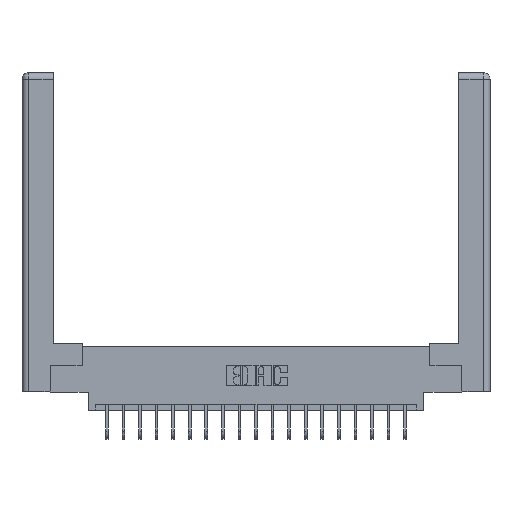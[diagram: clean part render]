
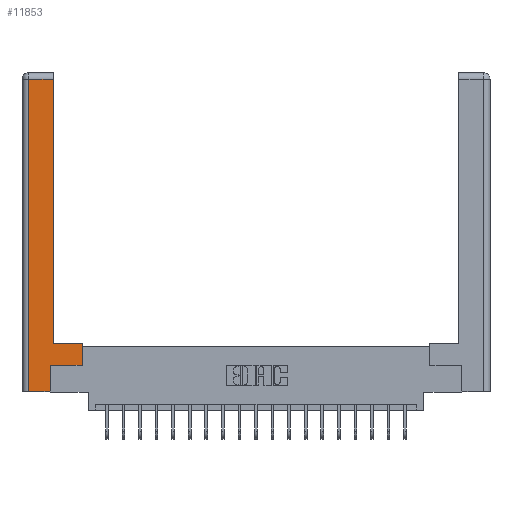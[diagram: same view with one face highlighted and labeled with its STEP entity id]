
A CAD part, top view. The second image highlights one B-rep face of the part: STEP entity #11853.
In plain terms, the highlighted planar face has unit normal (0, 0, 1).
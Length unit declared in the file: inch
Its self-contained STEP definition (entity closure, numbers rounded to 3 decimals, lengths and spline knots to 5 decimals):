
#339 = ORIENTED_EDGE ( 'NONE', *, *, #3760, .T. ) ;
#379 = ORIENTED_EDGE ( 'NONE', *, *, #7342, .T. ) ;
#838 = LINE ( 'NONE', #19871, #16722 ) ;
#1126 = DIRECTION ( 'NONE',  ( 0., 1., 0. ) ) ;
#1368 = VECTOR ( 'NONE', #1126, 39.37008 ) ;
#1410 = CARTESIAN_POINT ( 'NONE',  ( 0.265, 0., 0. ) ) ;
#1570 = DIRECTION ( 'NONE',  ( 0., -1., 0. ) ) ;
#1573 = DIRECTION ( 'NONE',  ( 0., 0., -1. ) ) ;
#1800 = CARTESIAN_POINT ( 'NONE',  ( 0.295, 2.94, 0. ) ) ;
#2307 = VECTOR ( 'NONE', #7888, 39.37008 ) ;
#2729 = VERTEX_POINT ( 'NONE', #1410 ) ;
#2953 = PLANE ( 'NONE',  #9144 ) ;
#3264 = VERTEX_POINT ( 'NONE', #1800 ) ;
#3324 = ORIENTED_EDGE ( 'NONE', *, *, #17834, .T. ) ;
#3383 = CARTESIAN_POINT ( 'NONE',  ( 0.0615, 2.94, 0. ) ) ;
#3439 = DIRECTION ( 'NONE',  ( -1., 0., 0. ) ) ;
#3760 = EDGE_CURVE ( 'NONE', #2729, #11741, #12435, .T. ) ;
#4003 = LINE ( 'NONE', #11118, #6613 ) ;
#4198 = ORIENTED_EDGE ( 'NONE', *, *, #4895, .T. ) ;
#4302 = CARTESIAN_POINT ( 'NONE',  ( 0.565, 0.45, 0. ) ) ;
#4895 = EDGE_CURVE ( 'NONE', #11741, #9619, #16220, .T. ) ;
#5053 = VECTOR ( 'NONE', #18982, 39.37008 ) ;
#5098 = ORIENTED_EDGE ( 'NONE', *, *, #16155, .T. ) ;
#5100 = EDGE_LOOP ( 'NONE', ( #3324, #5098, #17034, #9312, #339, #4198, #379, #8894 ) ) ;
#6091 = CARTESIAN_POINT ( 'NONE',  ( 0.565, 0.245, 0. ) ) ;
#6613 = VECTOR ( 'NONE', #3439, 39.37008 ) ;
#7342 = EDGE_CURVE ( 'NONE', #9619, #14809, #18332, .T. ) ;
#7733 = CARTESIAN_POINT ( 'NONE',  ( 0.295, 0.45, 0. ) ) ;
#7794 = VECTOR ( 'NONE', #10192, 39.37008 ) ;
#7857 = FACE_OUTER_BOUND ( 'NONE', #5100, .T. ) ;
#7888 = DIRECTION ( 'NONE',  ( -1., 0., 0. ) ) ;
#8385 = CARTESIAN_POINT ( 'NONE',  ( 0.565, 0.45, 0. ) ) ;
#8749 = CARTESIAN_POINT ( 'NONE',  ( 0.0615, 2.94, 0. ) ) ;
#8894 = ORIENTED_EDGE ( 'NONE', *, *, #11958, .T. ) ;
#8956 = VERTEX_POINT ( 'NONE', #8749 ) ;
#9144 = AXIS2_PLACEMENT_3D ( 'NONE', #19874, #1573, #19805 ) ;
#9312 = ORIENTED_EDGE ( 'NONE', *, *, #19507, .T. ) ;
#9619 = VERTEX_POINT ( 'NONE', #6091 ) ;
#9929 = VECTOR ( 'NONE', #19570, 39.37008 ) ;
#10192 = DIRECTION ( 'NONE',  ( 1., 0., 0. ) ) ;
#10318 = CARTESIAN_POINT ( 'NONE',  ( 0.265, 0.245, 0. ) ) ;
#10457 = CARTESIAN_POINT ( 'NONE',  ( 0.265, 0.245, 0. ) ) ;
#11118 = CARTESIAN_POINT ( 'NONE',  ( 0.295, 0.45, 0. ) ) ;
#11140 = VERTEX_POINT ( 'NONE', #13622 ) ;
#11232 = CARTESIAN_POINT ( 'NONE',  ( 0.265, 0., 0. ) ) ;
#11741 = VERTEX_POINT ( 'NONE', #10318 ) ;
#11853 = ADVANCED_FACE ( 'NONE', ( #7857 ), #2953, .F. ) ;
#11958 = EDGE_CURVE ( 'NONE', #14809, #15805, #4003, .T. ) ;
#12435 = LINE ( 'NONE', #10457, #1368 ) ;
#12855 = EDGE_CURVE ( 'NONE', #8956, #11140, #838, .T. ) ;
#13622 = CARTESIAN_POINT ( 'NONE',  ( 0.0615, 0., 0. ) ) ;
#13854 = LINE ( 'NONE', #3383, #2307 ) ;
#14809 = VERTEX_POINT ( 'NONE', #8385 ) ;
#15131 = DIRECTION ( 'NONE',  ( 0., 1., 0. ) ) ;
#15805 = VERTEX_POINT ( 'NONE', #7733 ) ;
#16155 = EDGE_CURVE ( 'NONE', #3264, #8956, #13854, .T. ) ;
#16220 = LINE ( 'NONE', #19562, #7794 ) ;
#16722 = VECTOR ( 'NONE', #1570, 39.37008 ) ;
#17034 = ORIENTED_EDGE ( 'NONE', *, *, #12855, .T. ) ;
#17808 = LINE ( 'NONE', #11232, #5053 ) ;
#17834 = EDGE_CURVE ( 'NONE', #15805, #3264, #18114, .T. ) ;
#18011 = CARTESIAN_POINT ( 'NONE',  ( 0.295, 3., 0. ) ) ;
#18114 = LINE ( 'NONE', #18011, #9929 ) ;
#18332 = LINE ( 'NONE', #4302, #19777 ) ;
#18982 = DIRECTION ( 'NONE',  ( 1., 0., 0. ) ) ;
#19507 = EDGE_CURVE ( 'NONE', #11140, #2729, #17808, .T. ) ;
#19562 = CARTESIAN_POINT ( 'NONE',  ( 0.565, 0.245, 0. ) ) ;
#19570 = DIRECTION ( 'NONE',  ( 0., 1., 0. ) ) ;
#19777 = VECTOR ( 'NONE', #15131, 39.37008 ) ;
#19805 = DIRECTION ( 'NONE',  ( -1., 0., 0. ) ) ;
#19871 = CARTESIAN_POINT ( 'NONE',  ( 0.0615, 0., 0. ) ) ;
#19874 = CARTESIAN_POINT ( 'NONE',  ( 0., 0., 0. ) ) ;
